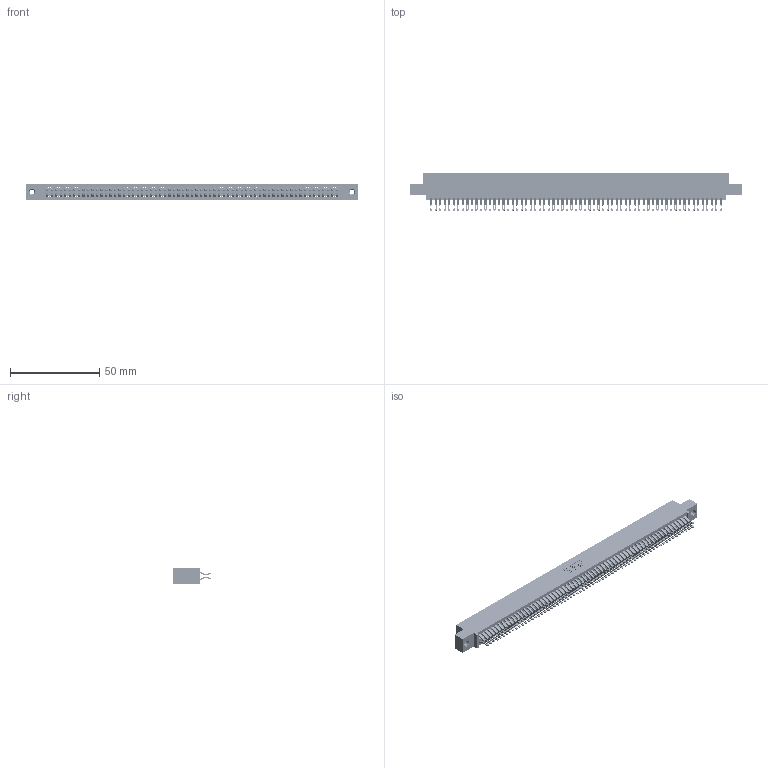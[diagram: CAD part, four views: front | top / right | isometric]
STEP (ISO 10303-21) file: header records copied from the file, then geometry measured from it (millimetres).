
FILE_DESCRIPTION (( 'STEP AP203' ), '1' );
FILE_NAME ('345-130-555-507.STEP', '2019-11-07T15:32:59', ( '' ), ( '' ), 'SwSTEP 2.0', 'SolidWorks 2016', '' );
FILE_SCHEMA (( 'CONFIG_CONTROL_DESIGN' ));
Length unit declared in the file: inch
Products named in the file (4): 345 Part_0.110 Offset - 0.156 Dia-TI; 345-250-001_345-250-005-103; 345-292-001_555 Tail; 345-130-555-507
Assembly tree (133 placements, depth 2):
  345-130-555-507
    345 Part_0.110 Offset - 0.156 Dia-TI
    345-292-001_555 Tail  x130
    345-250-001_345-250-005-103  x2
Bounding box: 186.31 x 21.13 x 9.4 mm (x, y, z)
Volume: 18601.9 mm3; surface area: 29374.4 mm2
Topology: 133 solids, 133 shells, 7470 faces, 23499 edges, 15658 vertices
Faces by surface type: plane 4146, cylinder 3308, cone 12, torus 4
Entity records: 49548 total; most frequent: CARTESIAN_POINT 8301, ORIENTED_EDGE 8198, DIRECTION 7285, EDGE_CURVE 4099, VECTOR 3667, LINE 3667, VERTEX_POINT 2728, AXIS2_PLACEMENT_3D 1809
